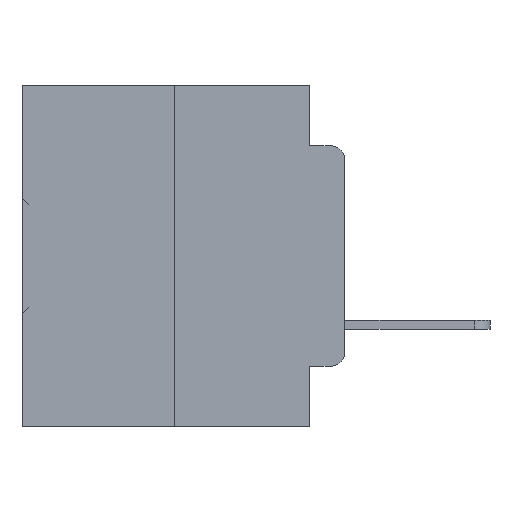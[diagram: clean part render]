
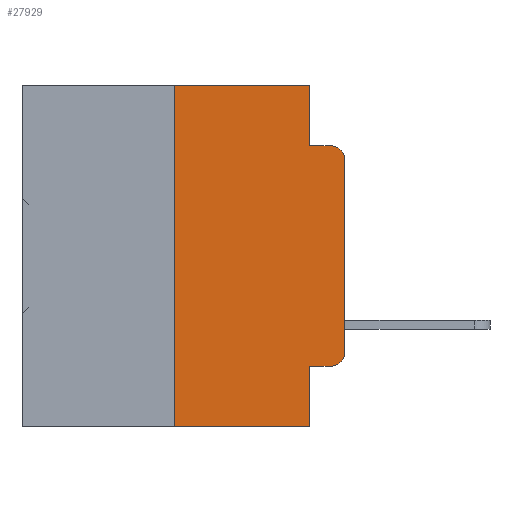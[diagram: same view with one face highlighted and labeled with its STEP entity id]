
A CAD part, left-side view. The second image highlights one B-rep face of the part: STEP entity #27929.
In plain terms, the highlighted planar face has unit normal (-1, 0, 0).
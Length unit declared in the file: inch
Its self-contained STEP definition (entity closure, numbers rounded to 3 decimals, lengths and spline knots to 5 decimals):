
#992 = EDGE_LOOP ( 'NONE', ( #16147, #35587, #23094, #24326, #6715, #20468, #22910, #24942, #27670, #30262 ) ) ;
#1780 = DIRECTION ( 'NONE',  ( 0., 0., 1. ) ) ;
#1957 = EDGE_CURVE ( 'NONE', #6092, #23288, #30881, .T. ) ;
#2009 = DIRECTION ( 'NONE',  ( -1., 0., 0. ) ) ;
#2692 = EDGE_CURVE ( 'NONE', #8665, #36192, #30884, .T. ) ;
#3034 = LINE ( 'NONE', #35203, #10191 ) ;
#3244 = DIRECTION ( 'NONE',  ( 0., -1., 0. ) ) ;
#3697 = CARTESIAN_POINT ( 'NONE',  ( 0., 0.051, 0. ) ) ;
#4748 = CARTESIAN_POINT ( 'NONE',  ( 0., 0.051, -0.4115 ) ) ;
#5199 = EDGE_CURVE ( 'NONE', #9094, #20350, #28705, .T. ) ;
#5466 = VECTOR ( 'NONE', #21245, 39.37008 ) ;
#6067 = AXIS2_PLACEMENT_3D ( 'NONE', #36112, #27330, #24111 ) ;
#6092 = VERTEX_POINT ( 'NONE', #28907 ) ;
#6357 = LINE ( 'NONE', #35537, #13539 ) ;
#6715 = ORIENTED_EDGE ( 'NONE', *, *, #5199, .F. ) ;
#7366 = LINE ( 'NONE', #9611, #5466 ) ;
#8034 = EDGE_CURVE ( 'NONE', #26687, #9094, #7366, .T. ) ;
#8665 = VERTEX_POINT ( 'NONE', #12776 ) ;
#9094 = VERTEX_POINT ( 'NONE', #20690 ) ;
#9611 = CARTESIAN_POINT ( 'NONE',  ( 0., 0.25, 0. ) ) ;
#10191 = VECTOR ( 'NONE', #1780, 39.37008 ) ;
#10618 = EDGE_CURVE ( 'NONE', #36192, #20286, #3034, .T. ) ;
#11132 = LINE ( 'NONE', #33173, #23508 ) ;
#11349 = CIRCLE ( 'NONE', #32540, 0.02 ) ;
#11630 = FACE_OUTER_BOUND ( 'NONE', #992, .T. ) ;
#11646 = LINE ( 'NONE', #4748, #27319 ) ;
#12776 = CARTESIAN_POINT ( 'NONE',  ( 0., 0.02, -0.4115 ) ) ;
#13539 = VECTOR ( 'NONE', #25199, 39.37008 ) ;
#14189 = VERTEX_POINT ( 'NONE', #30733 ) ;
#14472 = AXIS2_PLACEMENT_3D ( 'NONE', #28543, #31134, #15056 ) ;
#15056 = DIRECTION ( 'NONE',  ( 0., 0., -1. ) ) ;
#15406 = EDGE_CURVE ( 'NONE', #17155, #14189, #28673, .T. ) ;
#16147 = ORIENTED_EDGE ( 'NONE', *, *, #10618, .T. ) ;
#17155 = VERTEX_POINT ( 'NONE', #25943 ) ;
#17707 = CARTESIAN_POINT ( 'NONE',  ( 0., 0.25, -0.5 ) ) ;
#18150 = CARTESIAN_POINT ( 'NONE',  ( 0., 0.051, -0.0885 ) ) ;
#18328 = CARTESIAN_POINT ( 'NONE',  ( 0., 0., -0.1085 ) ) ;
#18519 = EDGE_CURVE ( 'NONE', #26687, #23288, #6357, .T. ) ;
#19122 = DIRECTION ( 'NONE',  ( 0., -1., 0. ) ) ;
#19276 = CARTESIAN_POINT ( 'NONE',  ( 0., 0.473, 0. ) ) ;
#19774 = CARTESIAN_POINT ( 'NONE',  ( 0., 0.02, -0.1085 ) ) ;
#20286 = VERTEX_POINT ( 'NONE', #18328 ) ;
#20350 = VERTEX_POINT ( 'NONE', #3697 ) ;
#20468 = ORIENTED_EDGE ( 'NONE', *, *, #8034, .F. ) ;
#20526 = EDGE_CURVE ( 'NONE', #6092, #8665, #11646, .T. ) ;
#20690 = CARTESIAN_POINT ( 'NONE',  ( 0., 0.25, 0. ) ) ;
#21245 = DIRECTION ( 'NONE',  ( 0., 0., 1. ) ) ;
#22331 = CARTESIAN_POINT ( 'NONE',  ( 0., 0.051, 0. ) ) ;
#22490 = DIRECTION ( 'NONE',  ( 0., 0., -1. ) ) ;
#22845 = DIRECTION ( 'NONE',  ( 0., 0., -1. ) ) ;
#22910 = ORIENTED_EDGE ( 'NONE', *, *, #18519, .T. ) ;
#23094 = ORIENTED_EDGE ( 'NONE', *, *, #15406, .F. ) ;
#23225 = PLANE ( 'NONE',  #14472 ) ;
#23288 = VERTEX_POINT ( 'NONE', #29802 ) ;
#23508 = VECTOR ( 'NONE', #22845, 39.37008 ) ;
#24111 = DIRECTION ( 'NONE',  ( 0., 0., -1. ) ) ;
#24326 = ORIENTED_EDGE ( 'NONE', *, *, #28761, .F. ) ;
#24911 = DIRECTION ( 'NONE',  ( 0., -1., 0. ) ) ;
#24942 = ORIENTED_EDGE ( 'NONE', *, *, #1957, .F. ) ;
#25199 = DIRECTION ( 'NONE',  ( 0., -1., 0. ) ) ;
#25943 = CARTESIAN_POINT ( 'NONE',  ( 0., 0.051, -0.0885 ) ) ;
#26687 = VERTEX_POINT ( 'NONE', #17707 ) ;
#27319 = VECTOR ( 'NONE', #24911, 39.37008 ) ;
#27330 = DIRECTION ( 'NONE',  ( -1., 0., 0. ) ) ;
#27670 = ORIENTED_EDGE ( 'NONE', *, *, #20526, .T. ) ;
#27881 = VECTOR ( 'NONE', #3244, 39.37008 ) ;
#27929 = ADVANCED_FACE ( 'NONE', ( #11630 ), #23225, .F. ) ;
#28543 = CARTESIAN_POINT ( 'NONE',  ( 0., 0.473, 0. ) ) ;
#28673 = LINE ( 'NONE', #18150, #27881 ) ;
#28705 = LINE ( 'NONE', #19276, #35466 ) ;
#28761 = EDGE_CURVE ( 'NONE', #20350, #17155, #11132, .T. ) ;
#28907 = CARTESIAN_POINT ( 'NONE',  ( 0., 0.051, -0.4115 ) ) ;
#29802 = CARTESIAN_POINT ( 'NONE',  ( 0., 0.051, -0.5 ) ) ;
#30078 = VECTOR ( 'NONE', #34468, 39.37008 ) ;
#30262 = ORIENTED_EDGE ( 'NONE', *, *, #2692, .T. ) ;
#30733 = CARTESIAN_POINT ( 'NONE',  ( 0., 0.02, -0.0885 ) ) ;
#30881 = LINE ( 'NONE', #22331, #30078 ) ;
#30884 = CIRCLE ( 'NONE', #6067, 0.02 ) ;
#31134 = DIRECTION ( 'NONE',  ( 1., 0., 0. ) ) ;
#32540 = AXIS2_PLACEMENT_3D ( 'NONE', #19774, #2009, #22490 ) ;
#33173 = CARTESIAN_POINT ( 'NONE',  ( 0., 0.051, 0. ) ) ;
#34093 = CARTESIAN_POINT ( 'NONE',  ( 0., 0., -0.3915 ) ) ;
#34468 = DIRECTION ( 'NONE',  ( 0., 0., -1. ) ) ;
#34927 = EDGE_CURVE ( 'NONE', #20286, #14189, #11349, .T. ) ;
#35203 = CARTESIAN_POINT ( 'NONE',  ( 0., 0., 0. ) ) ;
#35466 = VECTOR ( 'NONE', #19122, 39.37008 ) ;
#35537 = CARTESIAN_POINT ( 'NONE',  ( 0., 0.473, -0.5 ) ) ;
#35587 = ORIENTED_EDGE ( 'NONE', *, *, #34927, .T. ) ;
#36112 = CARTESIAN_POINT ( 'NONE',  ( 0., 0.02, -0.3915 ) ) ;
#36192 = VERTEX_POINT ( 'NONE', #34093 ) ;
